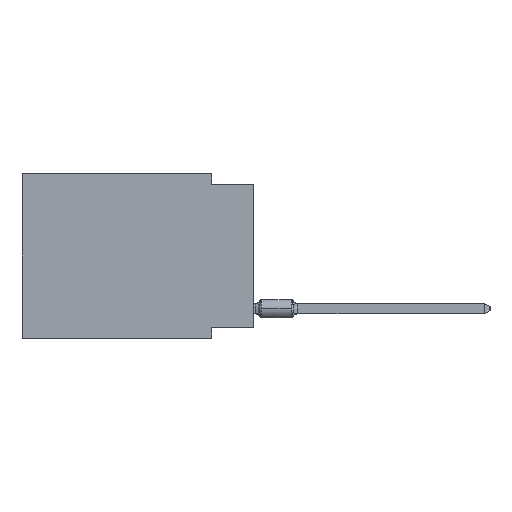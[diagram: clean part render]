
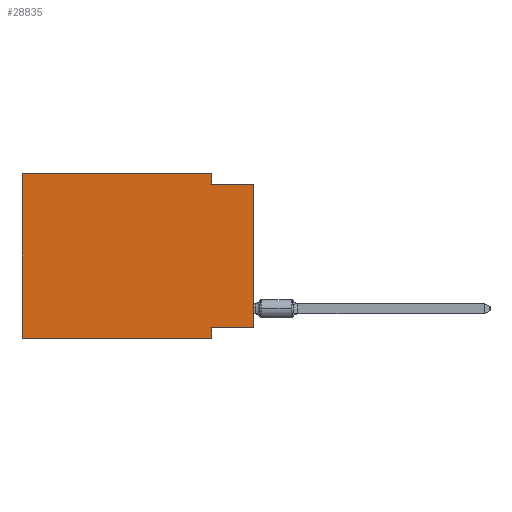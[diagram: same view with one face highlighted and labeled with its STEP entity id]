
A CAD part, left-side view. The second image highlights one B-rep face of the part: STEP entity #28835.
In plain terms, the highlighted planar face has unit normal (-1, 0, 0).
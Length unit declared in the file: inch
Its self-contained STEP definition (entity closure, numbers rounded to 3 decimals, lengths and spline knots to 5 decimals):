
#1215 = CARTESIAN_POINT ( 'NONE',  ( 0., 0.1, -0.365 ) ) ;
#1661 = VECTOR ( 'NONE', #2359, 39.37008 ) ;
#2047 = EDGE_CURVE ( 'NONE', #6457, #10323, #15708, .T. ) ;
#2359 = DIRECTION ( 'NONE',  ( 0., 0., 1. ) ) ;
#3789 = AXIS2_PLACEMENT_3D ( 'NONE', #18744, #35863, #7600 ) ;
#4620 = VERTEX_POINT ( 'NONE', #14581 ) ;
#5292 = VECTOR ( 'NONE', #33954, 39.37008 ) ;
#5455 = CARTESIAN_POINT ( 'NONE',  ( 0., 0.55, 0. ) ) ;
#5814 = VERTEX_POINT ( 'NONE', #12329 ) ;
#6393 = LINE ( 'NONE', #34126, #5292 ) ;
#6457 = VERTEX_POINT ( 'NONE', #32721 ) ;
#6657 = CARTESIAN_POINT ( 'NONE',  ( 0., 0.55, 0. ) ) ;
#6736 = EDGE_CURVE ( 'NONE', #10323, #22735, #21559, .T. ) ;
#6937 = VECTOR ( 'NONE', #35997, 39.37008 ) ;
#7600 = DIRECTION ( 'NONE',  ( 0., 0., -1. ) ) ;
#7643 = ORIENTED_EDGE ( 'NONE', *, *, #21760, .F. ) ;
#8062 = CARTESIAN_POINT ( 'NONE',  ( 0., 0.1, 0. ) ) ;
#9341 = VECTOR ( 'NONE', #32415, 39.37008 ) ;
#10323 = VERTEX_POINT ( 'NONE', #6657 ) ;
#10758 = DIRECTION ( 'NONE',  ( 0., -1., 0. ) ) ;
#11045 = FACE_OUTER_BOUND ( 'NONE', #36046, .T. ) ;
#11655 = ORIENTED_EDGE ( 'NONE', *, *, #2047, .F. ) ;
#12329 = CARTESIAN_POINT ( 'NONE',  ( 0., 0.1, -0.025 ) ) ;
#12900 = ORIENTED_EDGE ( 'NONE', *, *, #35092, .T. ) ;
#14474 = EDGE_CURVE ( 'NONE', #6457, #18396, #29814, .T. ) ;
#14581 = CARTESIAN_POINT ( 'NONE',  ( 0., 0., -0.365 ) ) ;
#14917 = CARTESIAN_POINT ( 'NONE',  ( 0., 0.1, -0.39 ) ) ;
#15708 = LINE ( 'NONE', #18978, #1661 ) ;
#15865 = ORIENTED_EDGE ( 'NONE', *, *, #6736, .F. ) ;
#16370 = ORIENTED_EDGE ( 'NONE', *, *, #14474, .T. ) ;
#18206 = ORIENTED_EDGE ( 'NONE', *, *, #28412, .F. ) ;
#18396 = VERTEX_POINT ( 'NONE', #28329 ) ;
#18744 = CARTESIAN_POINT ( 'NONE',  ( 0., 0.55, 0. ) ) ;
#18818 = EDGE_CURVE ( 'NONE', #22735, #5814, #6393, .T. ) ;
#18978 = CARTESIAN_POINT ( 'NONE',  ( 0., 0.55, 0. ) ) ;
#19099 = CARTESIAN_POINT ( 'NONE',  ( 0., 0., -0.025 ) ) ;
#19285 = VECTOR ( 'NONE', #20952, 39.37008 ) ;
#19865 = ORIENTED_EDGE ( 'NONE', *, *, #18818, .F. ) ;
#20952 = DIRECTION ( 'NONE',  ( 0., 0., -1. ) ) ;
#21142 = CARTESIAN_POINT ( 'NONE',  ( 0., 0., -0.365 ) ) ;
#21559 = LINE ( 'NONE', #5455, #30780 ) ;
#21660 = LINE ( 'NONE', #19099, #35901 ) ;
#21760 = EDGE_CURVE ( 'NONE', #28713, #18396, #34994, .T. ) ;
#21825 = DIRECTION ( 'NONE',  ( 0., -1., 0. ) ) ;
#22735 = VERTEX_POINT ( 'NONE', #8062 ) ;
#24238 = DIRECTION ( 'NONE',  ( 0., 1., 0. ) ) ;
#25802 = ORIENTED_EDGE ( 'NONE', *, *, #30065, .F. ) ;
#28329 = CARTESIAN_POINT ( 'NONE',  ( 0., 0.1, -0.39 ) ) ;
#28412 = EDGE_CURVE ( 'NONE', #4620, #28713, #29178, .T. ) ;
#28713 = VERTEX_POINT ( 'NONE', #1215 ) ;
#28835 = ADVANCED_FACE ( 'NONE', ( #11045 ), #32600, .F. ) ;
#29178 = LINE ( 'NONE', #21142, #30003 ) ;
#29496 = LINE ( 'NONE', #34798, #9341 ) ;
#29814 = LINE ( 'NONE', #30349, #6937 ) ;
#30003 = VECTOR ( 'NONE', #24238, 39.37008 ) ;
#30065 = EDGE_CURVE ( 'NONE', #5814, #35229, #21660, .T. ) ;
#30349 = CARTESIAN_POINT ( 'NONE',  ( 0., 0.55, -0.39 ) ) ;
#30780 = VECTOR ( 'NONE', #10758, 39.37008 ) ;
#32415 = DIRECTION ( 'NONE',  ( 0., 0., 1. ) ) ;
#32600 = PLANE ( 'NONE',  #3789 ) ;
#32721 = CARTESIAN_POINT ( 'NONE',  ( 0., 0.55, -0.39 ) ) ;
#33954 = DIRECTION ( 'NONE',  ( 0., 0., -1. ) ) ;
#34126 = CARTESIAN_POINT ( 'NONE',  ( 0., 0.1, 0. ) ) ;
#34798 = CARTESIAN_POINT ( 'NONE',  ( 0., 0., 0. ) ) ;
#34994 = LINE ( 'NONE', #14917, #19285 ) ;
#35092 = EDGE_CURVE ( 'NONE', #4620, #35229, #29496, .T. ) ;
#35229 = VERTEX_POINT ( 'NONE', #35334 ) ;
#35334 = CARTESIAN_POINT ( 'NONE',  ( 0., 0., -0.025 ) ) ;
#35863 = DIRECTION ( 'NONE',  ( 1., 0., 0. ) ) ;
#35901 = VECTOR ( 'NONE', #21825, 39.37008 ) ;
#35997 = DIRECTION ( 'NONE',  ( 0., -1., 0. ) ) ;
#36046 = EDGE_LOOP ( 'NONE', ( #12900, #25802, #19865, #15865, #11655, #16370, #7643, #18206 ) ) ;
